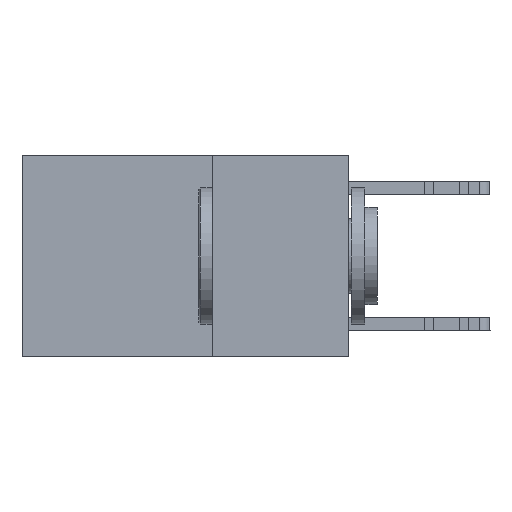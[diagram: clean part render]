
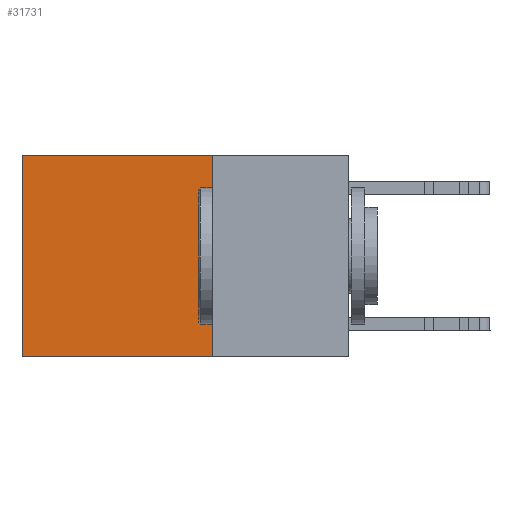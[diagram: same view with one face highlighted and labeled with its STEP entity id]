
A CAD part, left-side view. The second image highlights one B-rep face of the part: STEP entity #31731.
In plain terms, the highlighted planar face has unit normal (-1, 0, 0).
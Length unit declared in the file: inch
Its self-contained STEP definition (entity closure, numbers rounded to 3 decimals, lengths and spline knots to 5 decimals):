
#2348 = ORIENTED_EDGE ( 'NONE', *, *, #28722, .F. ) ;
#3568 = FACE_OUTER_BOUND ( 'NONE', #8305, .T. ) ;
#3728 = CARTESIAN_POINT ( 'NONE',  ( 0.2625, 0.25, 0. ) ) ;
#3922 = VERTEX_POINT ( 'NONE', #22375 ) ;
#3971 = DIRECTION ( 'NONE',  ( 0., 1., 0. ) ) ;
#4129 = DIRECTION ( 'NONE',  ( 0., 1., 0. ) ) ;
#4691 = CARTESIAN_POINT ( 'NONE',  ( 0.2625, 0.25, 0. ) ) ;
#5603 = CARTESIAN_POINT ( 'NONE',  ( 0.2625, 0.6, -0.37 ) ) ;
#6319 = EDGE_CURVE ( 'NONE', #7143, #19639, #19207, .T. ) ;
#7143 = VERTEX_POINT ( 'NONE', #22861 ) ;
#7208 = ORIENTED_EDGE ( 'NONE', *, *, #16850, .T. ) ;
#7494 = LINE ( 'NONE', #12211, #24637 ) ;
#8305 = EDGE_LOOP ( 'NONE', ( #7208, #18995, #2348, #25891 ) ) ;
#8770 = DIRECTION ( 'NONE',  ( 0., 0., -1. ) ) ;
#12211 = CARTESIAN_POINT ( 'NONE',  ( 0.2625, 0.6, 0. ) ) ;
#14916 = EDGE_CURVE ( 'NONE', #3922, #23259, #21156, .T. ) ;
#15075 = CARTESIAN_POINT ( 'NONE',  ( 0.2625, 0.6, 0. ) ) ;
#16619 = CARTESIAN_POINT ( 'NONE',  ( 0.2625, 0.25, -0.37 ) ) ;
#16850 = EDGE_CURVE ( 'NONE', #19639, #23259, #7494, .T. ) ;
#18337 = PLANE ( 'NONE',  #26575 ) ;
#18995 = ORIENTED_EDGE ( 'NONE', *, *, #14916, .F. ) ;
#19193 = VECTOR ( 'NONE', #24452, 39.37008 ) ;
#19207 = LINE ( 'NONE', #21475, #21471 ) ;
#19593 = LINE ( 'NONE', #4691, #19193 ) ;
#19639 = VERTEX_POINT ( 'NONE', #15075 ) ;
#21156 = LINE ( 'NONE', #16619, #29768 ) ;
#21471 = VECTOR ( 'NONE', #4129, 39.37008 ) ;
#21475 = CARTESIAN_POINT ( 'NONE',  ( 0.2625, 0.25, 0. ) ) ;
#22375 = CARTESIAN_POINT ( 'NONE',  ( 0.2625, 0.25, -0.37 ) ) ;
#22861 = CARTESIAN_POINT ( 'NONE',  ( 0.2625, 0.25, 0. ) ) ;
#23259 = VERTEX_POINT ( 'NONE', #5603 ) ;
#24452 = DIRECTION ( 'NONE',  ( 0., 0., -1. ) ) ;
#24637 = VECTOR ( 'NONE', #29398, 39.37008 ) ;
#25891 = ORIENTED_EDGE ( 'NONE', *, *, #6319, .T. ) ;
#26575 = AXIS2_PLACEMENT_3D ( 'NONE', #3728, #28235, #8770 ) ;
#28235 = DIRECTION ( 'NONE',  ( 1., 0., 0. ) ) ;
#28722 = EDGE_CURVE ( 'NONE', #7143, #3922, #19593, .T. ) ;
#29398 = DIRECTION ( 'NONE',  ( 0., 0., -1. ) ) ;
#29768 = VECTOR ( 'NONE', #3971, 39.37008 ) ;
#31731 = ADVANCED_FACE ( 'NONE', ( #3568 ), #18337, .F. ) ;
